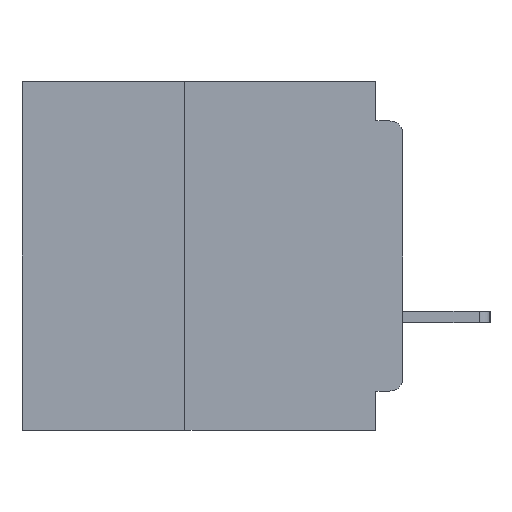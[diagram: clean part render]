
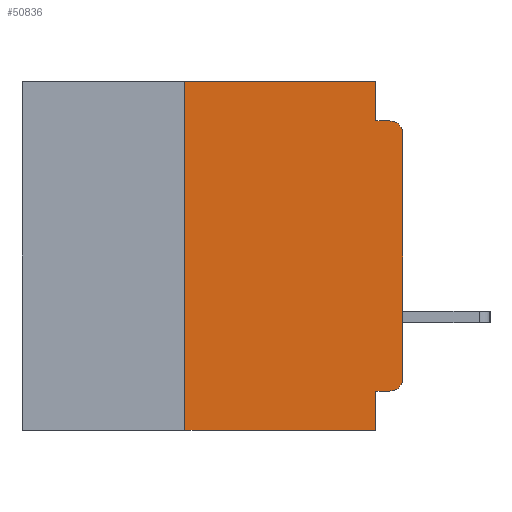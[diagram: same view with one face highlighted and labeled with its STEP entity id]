
A CAD part, left-side view. The second image highlights one B-rep face of the part: STEP entity #50836.
In plain terms, the highlighted planar face has unit normal (-1, 0, 0).
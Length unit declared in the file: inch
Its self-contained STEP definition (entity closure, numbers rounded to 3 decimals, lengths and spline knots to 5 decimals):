
#1039 = CARTESIAN_POINT ( 'NONE',  ( 0., 0.031, -0.4 ) ) ;
#2478 = VECTOR ( 'NONE', #22772, 39.37008 ) ;
#2665 = DIRECTION ( 'NONE',  ( 0., 0., -1. ) ) ;
#3641 = CARTESIAN_POINT ( 'NONE',  ( 0., 0.437, -0.4 ) ) ;
#4261 = CARTESIAN_POINT ( 'NONE',  ( 0., 0.25, -0.4 ) ) ;
#4933 = CARTESIAN_POINT ( 'NONE',  ( 0., 0.437, 0. ) ) ;
#6075 = VERTEX_POINT ( 'NONE', #34838 ) ;
#6567 = ORIENTED_EDGE ( 'NONE', *, *, #36922, .F. ) ;
#6585 = EDGE_CURVE ( 'NONE', #43050, #25166, #51494, .T. ) ;
#6699 = DIRECTION ( 'NONE',  ( 0., 0., -1. ) ) ;
#7228 = LINE ( 'NONE', #55524, #17164 ) ;
#7630 = ORIENTED_EDGE ( 'NONE', *, *, #26733, .F. ) ;
#8392 = DIRECTION ( 'NONE',  ( 0., -1., 0. ) ) ;
#9513 = VERTEX_POINT ( 'NONE', #26151 ) ;
#9770 = EDGE_CURVE ( 'NONE', #58419, #11356, #18430, .T. ) ;
#10348 = ORIENTED_EDGE ( 'NONE', *, *, #11745, .F. ) ;
#10477 = CARTESIAN_POINT ( 'NONE',  ( 0., 0.25, 0. ) ) ;
#10560 = LINE ( 'NONE', #17955, #23514 ) ;
#11356 = VERTEX_POINT ( 'NONE', #1039 ) ;
#11687 = ORIENTED_EDGE ( 'NONE', *, *, #6585, .F. ) ;
#11745 = EDGE_CURVE ( 'NONE', #58419, #43050, #54613, .T. ) ;
#12617 = VECTOR ( 'NONE', #46973, 39.37008 ) ;
#12715 = VECTOR ( 'NONE', #43903, 39.37008 ) ;
#13098 = CARTESIAN_POINT ( 'NONE',  ( 0., 0.25, -0.4 ) ) ;
#14603 = ORIENTED_EDGE ( 'NONE', *, *, #28564, .T. ) ;
#15202 = ORIENTED_EDGE ( 'NONE', *, *, #38208, .T. ) ;
#15843 = VECTOR ( 'NONE', #57660, 39.37008 ) ;
#16815 = CIRCLE ( 'NONE', #18699, 0.015 ) ;
#16880 = VECTOR ( 'NONE', #8392, 39.37008 ) ;
#17164 = VECTOR ( 'NONE', #36228, 39.37008 ) ;
#17955 = CARTESIAN_POINT ( 'NONE',  ( 0., 0., -0.045 ) ) ;
#18430 = LINE ( 'NONE', #3641, #16880 ) ;
#18517 = DIRECTION ( 'NONE',  ( 0., 1., 0. ) ) ;
#18699 = AXIS2_PLACEMENT_3D ( 'NONE', #27744, #61565, #32615 ) ;
#19486 = CARTESIAN_POINT ( 'NONE',  ( 0., 0.015, -0.355 ) ) ;
#21584 = EDGE_LOOP ( 'NONE', ( #14603, #27709, #7630, #6567, #11687, #10348, #52296, #52311, #26951, #15202 ) ) ;
#22772 = DIRECTION ( 'NONE',  ( 0., 0., -1. ) ) ;
#23514 = VECTOR ( 'NONE', #51931, 39.37008 ) ;
#23770 = VERTEX_POINT ( 'NONE', #39875 ) ;
#25166 = VERTEX_POINT ( 'NONE', #43214 ) ;
#26151 = CARTESIAN_POINT ( 'NONE',  ( 0., 0., -0.34 ) ) ;
#26164 = PLANE ( 'NONE',  #48905 ) ;
#26733 = EDGE_CURVE ( 'NONE', #6075, #38098, #10560, .T. ) ;
#26951 = ORIENTED_EDGE ( 'NONE', *, *, #60890, .F. ) ;
#27134 = LINE ( 'NONE', #37203, #12617 ) ;
#27709 = ORIENTED_EDGE ( 'NONE', *, *, #39605, .T. ) ;
#27744 = CARTESIAN_POINT ( 'NONE',  ( 0., 0.015, -0.34 ) ) ;
#28564 = EDGE_CURVE ( 'NONE', #9513, #23770, #7228, .T. ) ;
#31053 = CARTESIAN_POINT ( 'NONE',  ( 0., 0.437, 0. ) ) ;
#31788 = CARTESIAN_POINT ( 'NONE',  ( 0., 0.015, -0.045 ) ) ;
#31808 = VERTEX_POINT ( 'NONE', #19486 ) ;
#31956 = DIRECTION ( 'NONE',  ( -1., 0., 0. ) ) ;
#32615 = DIRECTION ( 'NONE',  ( 0., 0., -1. ) ) ;
#34838 = CARTESIAN_POINT ( 'NONE',  ( 0., 0.031, -0.045 ) ) ;
#35876 = DIRECTION ( 'NONE',  ( 1., 0., 0. ) ) ;
#36228 = DIRECTION ( 'NONE',  ( 0., 0., 1. ) ) ;
#36922 = EDGE_CURVE ( 'NONE', #25166, #6075, #27134, .T. ) ;
#37203 = CARTESIAN_POINT ( 'NONE',  ( 0., 0.031, 0. ) ) ;
#37606 = VERTEX_POINT ( 'NONE', #42628 ) ;
#38098 = VERTEX_POINT ( 'NONE', #31788 ) ;
#38208 = EDGE_CURVE ( 'NONE', #31808, #9513, #16815, .T. ) ;
#39605 = EDGE_CURVE ( 'NONE', #23770, #38098, #52364, .T. ) ;
#39875 = CARTESIAN_POINT ( 'NONE',  ( 0., 0., -0.06 ) ) ;
#42628 = CARTESIAN_POINT ( 'NONE',  ( 0., 0.031, -0.355 ) ) ;
#43050 = VERTEX_POINT ( 'NONE', #10477 ) ;
#43214 = CARTESIAN_POINT ( 'NONE',  ( 0., 0.031, 0. ) ) ;
#43903 = DIRECTION ( 'NONE',  ( 0., -1., 0. ) ) ;
#44472 = LINE ( 'NONE', #51869, #2478 ) ;
#46973 = DIRECTION ( 'NONE',  ( 0., 0., -1. ) ) ;
#48905 = AXIS2_PLACEMENT_3D ( 'NONE', #31053, #35876, #6699 ) ;
#49725 = LINE ( 'NONE', #57352, #62541 ) ;
#50836 = ADVANCED_FACE ( 'NONE', ( #60990 ), #26164, .F. ) ;
#51494 = LINE ( 'NONE', #4933, #12715 ) ;
#51869 = CARTESIAN_POINT ( 'NONE',  ( 0., 0.031, -0.4 ) ) ;
#51931 = DIRECTION ( 'NONE',  ( 0., -1., 0. ) ) ;
#52296 = ORIENTED_EDGE ( 'NONE', *, *, #9770, .T. ) ;
#52311 = ORIENTED_EDGE ( 'NONE', *, *, #60819, .F. ) ;
#52364 = CIRCLE ( 'NONE', #59363, 0.015 ) ;
#54613 = LINE ( 'NONE', #4261, #15843 ) ;
#55524 = CARTESIAN_POINT ( 'NONE',  ( 0., 0., 0. ) ) ;
#57352 = CARTESIAN_POINT ( 'NONE',  ( 0., 0., -0.355 ) ) ;
#57660 = DIRECTION ( 'NONE',  ( 0., 0., 1. ) ) ;
#58419 = VERTEX_POINT ( 'NONE', #13098 ) ;
#59363 = AXIS2_PLACEMENT_3D ( 'NONE', #60919, #31956, #2665 ) ;
#60819 = EDGE_CURVE ( 'NONE', #37606, #11356, #44472, .T. ) ;
#60890 = EDGE_CURVE ( 'NONE', #31808, #37606, #49725, .T. ) ;
#60919 = CARTESIAN_POINT ( 'NONE',  ( 0., 0.015, -0.06 ) ) ;
#60990 = FACE_OUTER_BOUND ( 'NONE', #21584, .T. ) ;
#61565 = DIRECTION ( 'NONE',  ( -1., 0., 0. ) ) ;
#62541 = VECTOR ( 'NONE', #18517, 39.37008 ) ;
